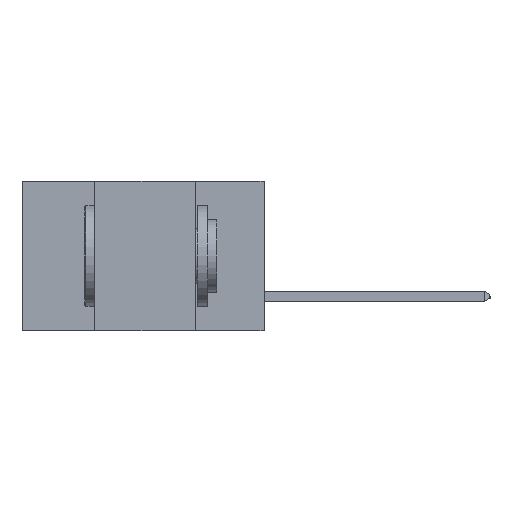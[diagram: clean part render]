
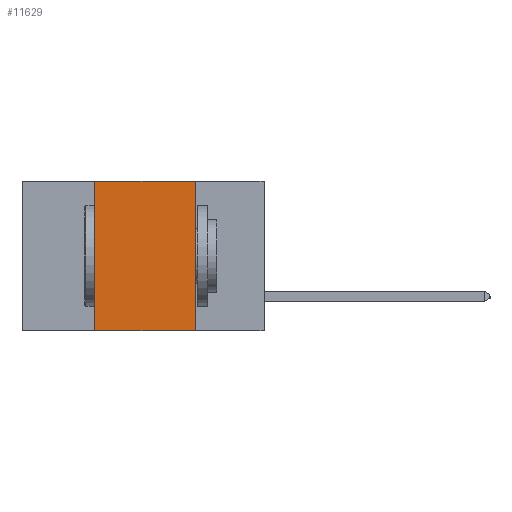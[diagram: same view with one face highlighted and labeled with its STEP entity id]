
A CAD part, left-side view. The second image highlights one B-rep face of the part: STEP entity #11629.
In plain terms, the highlighted planar face has unit normal (-1, 0, 0).
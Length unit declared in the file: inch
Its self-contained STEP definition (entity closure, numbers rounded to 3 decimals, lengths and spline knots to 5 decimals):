
#22 = CARTESIAN_POINT ( 'NONE',  ( 0., 0.42, 0. ) ) ;
#106 = VECTOR ( 'NONE', #6621, 39.37008 ) ;
#114 = VECTOR ( 'NONE', #4630, 39.37008 ) ;
#566 = LINE ( 'NONE', #22, #6288 ) ;
#839 = ORIENTED_EDGE ( 'NONE', *, *, #2846, .F. ) ;
#1349 = CARTESIAN_POINT ( 'NONE',  ( 0., 0.17, -0.37 ) ) ;
#1494 = ORIENTED_EDGE ( 'NONE', *, *, #6264, .F. ) ;
#1738 = CARTESIAN_POINT ( 'NONE',  ( 0., 0.6, 0. ) ) ;
#2846 = EDGE_CURVE ( 'NONE', #8739, #4938, #16672, .T. ) ;
#3879 = FACE_OUTER_BOUND ( 'NONE', #25746, .T. ) ;
#3920 = DIRECTION ( 'NONE',  ( 1., 0., 0. ) ) ;
#4516 = CARTESIAN_POINT ( 'NONE',  ( 0., 0.6, 0. ) ) ;
#4537 = CARTESIAN_POINT ( 'NONE',  ( 0., 0.17, 0. ) ) ;
#4630 = DIRECTION ( 'NONE',  ( 0., 0., -1. ) ) ;
#4938 = VERTEX_POINT ( 'NONE', #1349 ) ;
#6264 = EDGE_CURVE ( 'NONE', #22264, #12863, #566, .T. ) ;
#6288 = VECTOR ( 'NONE', #14616, 39.37008 ) ;
#6621 = DIRECTION ( 'NONE',  ( 0., -1., 0. ) ) ;
#6802 = CARTESIAN_POINT ( 'NONE',  ( 0., 0.17, 0. ) ) ;
#8739 = VERTEX_POINT ( 'NONE', #6802 ) ;
#10630 = LINE ( 'NONE', #4516, #106 ) ;
#11468 = DIRECTION ( 'NONE',  ( 0., -1., 0. ) ) ;
#11629 = ADVANCED_FACE ( 'NONE', ( #3879 ), #14162, .F. ) ;
#12863 = VERTEX_POINT ( 'NONE', #26267 ) ;
#14162 = PLANE ( 'NONE',  #22662 ) ;
#14439 = EDGE_CURVE ( 'NONE', #22264, #4938, #23644, .T. ) ;
#14616 = DIRECTION ( 'NONE',  ( 0., 0., 1. ) ) ;
#16672 = LINE ( 'NONE', #4537, #114 ) ;
#17458 = ORIENTED_EDGE ( 'NONE', *, *, #18781, .F. ) ;
#17487 = CARTESIAN_POINT ( 'NONE',  ( 0., 0.6, -0.37 ) ) ;
#18204 = DIRECTION ( 'NONE',  ( 0., 0., -1. ) ) ;
#18353 = VECTOR ( 'NONE', #11468, 39.37008 ) ;
#18781 = EDGE_CURVE ( 'NONE', #12863, #8739, #10630, .T. ) ;
#19250 = ORIENTED_EDGE ( 'NONE', *, *, #14439, .T. ) ;
#19985 = CARTESIAN_POINT ( 'NONE',  ( 0., 0.42, -0.37 ) ) ;
#22264 = VERTEX_POINT ( 'NONE', #19985 ) ;
#22662 = AXIS2_PLACEMENT_3D ( 'NONE', #1738, #3920, #18204 ) ;
#23644 = LINE ( 'NONE', #17487, #18353 ) ;
#25746 = EDGE_LOOP ( 'NONE', ( #839, #17458, #1494, #19250 ) ) ;
#26267 = CARTESIAN_POINT ( 'NONE',  ( 0., 0.42, 0. ) ) ;
